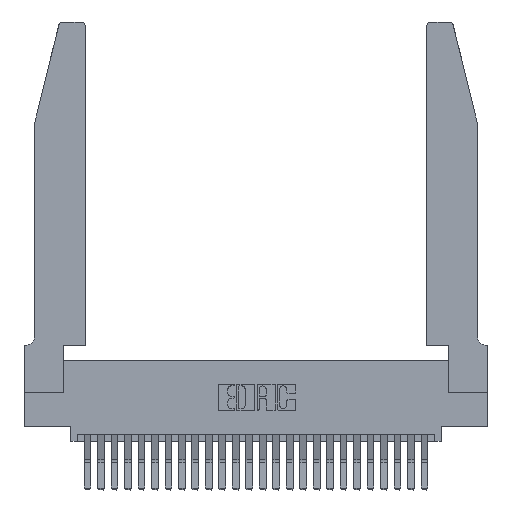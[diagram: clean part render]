
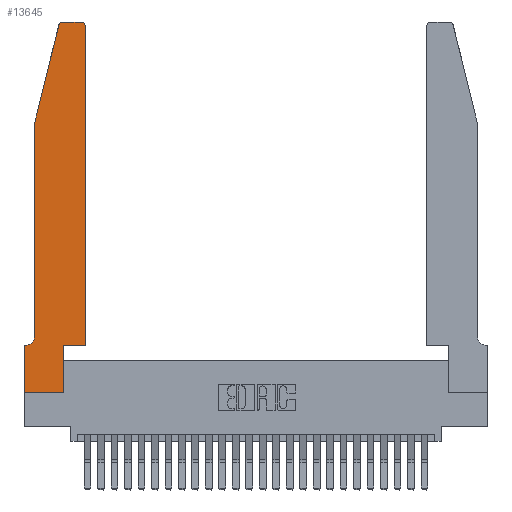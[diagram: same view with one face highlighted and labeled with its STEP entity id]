
A CAD part, top view. The second image highlights one B-rep face of the part: STEP entity #13645.
In plain terms, the highlighted planar face has unit normal (0, 0, 1).
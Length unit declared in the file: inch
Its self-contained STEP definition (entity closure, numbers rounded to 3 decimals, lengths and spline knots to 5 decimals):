
#191 = DIRECTION ( 'NONE',  ( -1., 0., 0. ) ) ;
#1623 = EDGE_CURVE ( 'NONE', #24799, #25691, #21712, .T. ) ;
#1647 = ORIENTED_EDGE ( 'NONE', *, *, #10541, .T. ) ;
#2577 = EDGE_CURVE ( 'NONE', #8014, #25782, #20995, .T. ) ;
#3032 = LINE ( 'NONE', #21042, #5004 ) ;
#3090 = CARTESIAN_POINT ( 'NONE',  ( 0.4505, 0.35, 0.37 ) ) ;
#3156 = EDGE_CURVE ( 'NONE', #8851, #26485, #5602, .T. ) ;
#3496 = DIRECTION ( 'NONE',  ( 1., 0., 0. ) ) ;
#3728 = VERTEX_POINT ( 'NONE', #27274 ) ;
#3862 = ORIENTED_EDGE ( 'NONE', *, *, #1623, .T. ) ;
#4601 = VECTOR ( 'NONE', #14679, 39.37008 ) ;
#4618 = CARTESIAN_POINT ( 'NONE',  ( 0.0055, 0.42, 0.37 ) ) ;
#5004 = VECTOR ( 'NONE', #8259, 39.37008 ) ;
#5112 = CARTESIAN_POINT ( 'NONE',  ( 0.2605, 2.75, 0.37 ) ) ;
#5154 = CARTESIAN_POINT ( 'NONE',  ( 0.0755, 2., 0.37 ) ) ;
#5415 = AXIS2_PLACEMENT_3D ( 'NONE', #16167, #5652, #9706 ) ;
#5602 = CIRCLE ( 'NONE', #13974, 0.07 ) ;
#5652 = DIRECTION ( 'NONE',  ( 0., 0., 1. ) ) ;
#5722 = CARTESIAN_POINT ( 'NONE',  ( 0.0755, 2., 0.37 ) ) ;
#5994 = CARTESIAN_POINT ( 'NONE',  ( 0., 0.35, 0.37 ) ) ;
#7004 = VECTOR ( 'NONE', #8012, 39.37008 ) ;
#7296 = EDGE_CURVE ( 'NONE', #27507, #11293, #3032, .T. ) ;
#7310 = CARTESIAN_POINT ( 'NONE',  ( 0.4205, 2.75, 0.37 ) ) ;
#7410 = DIRECTION ( 'NONE',  ( -0.239, -0.971, 0. ) ) ;
#8012 = DIRECTION ( 'NONE',  ( -1., 0., 0. ) ) ;
#8014 = VERTEX_POINT ( 'NONE', #7310 ) ;
#8026 = CARTESIAN_POINT ( 'NONE',  ( 0.0755, 2., 0.37 ) ) ;
#8071 = EDGE_CURVE ( 'NONE', #26485, #24799, #8670, .T. ) ;
#8141 = DIRECTION ( 'NONE',  ( 0., 1., 0. ) ) ;
#8259 = DIRECTION ( 'NONE',  ( 1., 0., 0. ) ) ;
#8312 = VECTOR ( 'NONE', #21281, 39.37008 ) ;
#8501 = CARTESIAN_POINT ( 'NONE',  ( 0., 0., 0.37 ) ) ;
#8670 = LINE ( 'NONE', #16443, #7004 ) ;
#8851 = VERTEX_POINT ( 'NONE', #23592 ) ;
#9061 = EDGE_CURVE ( 'NONE', #16507, #8851, #17365, .T. ) ;
#9536 = ORIENTED_EDGE ( 'NONE', *, *, #7296, .T. ) ;
#9549 = DIRECTION ( 'NONE',  ( 0., 1., 0. ) ) ;
#9706 = DIRECTION ( 'NONE',  ( 1., 0., 0. ) ) ;
#9871 = CARTESIAN_POINT ( 'NONE',  ( 0.4505, 2.72, 0.37 ) ) ;
#9877 = DIRECTION ( 'NONE',  ( 0., 0., 1. ) ) ;
#10463 = CARTESIAN_POINT ( 'NONE',  ( 0., 0., 0.37 ) ) ;
#10541 = EDGE_CURVE ( 'NONE', #11293, #24097, #25851, .T. ) ;
#11027 = ORIENTED_EDGE ( 'NONE', *, *, #16321, .T. ) ;
#11293 = VERTEX_POINT ( 'NONE', #25905 ) ;
#11529 = CARTESIAN_POINT ( 'NONE',  ( 0., 0., 0.37 ) ) ;
#12770 = EDGE_CURVE ( 'NONE', #24097, #8014, #15247, .T. ) ;
#13645 = ADVANCED_FACE ( 'NONE', ( #17851 ), #24749, .T. ) ;
#13974 = AXIS2_PLACEMENT_3D ( 'NONE', #4618, #17377, #191 ) ;
#14679 = DIRECTION ( 'NONE',  ( 0., -1., 0. ) ) ;
#15247 = CIRCLE ( 'NONE', #5415, 0.03 ) ;
#15413 = EDGE_LOOP ( 'NONE', ( #21035, #11027, #22888, #17339, #23902, #17139, #3862, #18591, #20110, #9536, #1647, #23882 ) ) ;
#16167 = CARTESIAN_POINT ( 'NONE',  ( 0.4205, 2.72, 0.37 ) ) ;
#16321 = EDGE_CURVE ( 'NONE', #25782, #16988, #19688, .T. ) ;
#16334 = CARTESIAN_POINT ( 'NONE',  ( 0., 0.35, 0.37 ) ) ;
#16443 = CARTESIAN_POINT ( 'NONE',  ( 0.0755, 0.35, 0.37 ) ) ;
#16507 = VERTEX_POINT ( 'NONE', #8026 ) ;
#16988 = VERTEX_POINT ( 'NONE', #22201 ) ;
#17003 = DIRECTION ( 'NONE',  ( 0., -1., 0. ) ) ;
#17102 = DIRECTION ( 'NONE',  ( 0., 0., 1. ) ) ;
#17139 = ORIENTED_EDGE ( 'NONE', *, *, #8071, .T. ) ;
#17339 = ORIENTED_EDGE ( 'NONE', *, *, #9061, .T. ) ;
#17363 = AXIS2_PLACEMENT_3D ( 'NONE', #16334, #9877, #3496 ) ;
#17365 = LINE ( 'NONE', #5722, #4601 ) ;
#17377 = DIRECTION ( 'NONE',  ( 0., 0., -1. ) ) ;
#17506 = VECTOR ( 'NONE', #7410, 39.37008 ) ;
#17851 = FACE_OUTER_BOUND ( 'NONE', #15413, .T. ) ;
#18591 = ORIENTED_EDGE ( 'NONE', *, *, #23031, .T. ) ;
#19032 = DIRECTION ( 'NONE',  ( 1., 0., 0. ) ) ;
#19242 = AXIS2_PLACEMENT_3D ( 'NONE', #21348, #17102, #19032 ) ;
#19688 = CIRCLE ( 'NONE', #19242, 0.03 ) ;
#19974 = LINE ( 'NONE', #27182, #20309 ) ;
#20110 = ORIENTED_EDGE ( 'NONE', *, *, #25981, .T. ) ;
#20244 = VECTOR ( 'NONE', #9549, 39.37008 ) ;
#20309 = VECTOR ( 'NONE', #8141, 39.37008 ) ;
#20372 = EDGE_CURVE ( 'NONE', #16988, #16507, #26743, .T. ) ;
#20995 = LINE ( 'NONE', #5112, #23967 ) ;
#21035 = ORIENTED_EDGE ( 'NONE', *, *, #2577, .T. ) ;
#21042 = CARTESIAN_POINT ( 'NONE',  ( 0.4505, 0.35, 0.37 ) ) ;
#21281 = DIRECTION ( 'NONE',  ( 1., 0., 0. ) ) ;
#21348 = CARTESIAN_POINT ( 'NONE',  ( 0.284, 2.72, 0.37 ) ) ;
#21712 = LINE ( 'NONE', #10463, #27008 ) ;
#22201 = CARTESIAN_POINT ( 'NONE',  ( 0.25487, 2.72718, 0.37 ) ) ;
#22577 = CARTESIAN_POINT ( 'NONE',  ( 0.0055, 0.35, 0.37 ) ) ;
#22888 = ORIENTED_EDGE ( 'NONE', *, *, #20372, .T. ) ;
#23031 = EDGE_CURVE ( 'NONE', #25691, #3728, #27268, .T. ) ;
#23592 = CARTESIAN_POINT ( 'NONE',  ( 0.0755, 0.42, 0.37 ) ) ;
#23882 = ORIENTED_EDGE ( 'NONE', *, *, #12770, .T. ) ;
#23902 = ORIENTED_EDGE ( 'NONE', *, *, #3156, .T. ) ;
#23967 = VECTOR ( 'NONE', #24408, 39.37008 ) ;
#24097 = VERTEX_POINT ( 'NONE', #9871 ) ;
#24408 = DIRECTION ( 'NONE',  ( -1., 0., 0. ) ) ;
#24427 = CARTESIAN_POINT ( 'NONE',  ( 0.284, 2.75, 0.37 ) ) ;
#24749 = PLANE ( 'NONE',  #17363 ) ;
#24799 = VERTEX_POINT ( 'NONE', #5994 ) ;
#25691 = VERTEX_POINT ( 'NONE', #11529 ) ;
#25782 = VERTEX_POINT ( 'NONE', #24427 ) ;
#25851 = LINE ( 'NONE', #3090, #20244 ) ;
#25905 = CARTESIAN_POINT ( 'NONE',  ( 0.4505, 0.35, 0.37 ) ) ;
#25981 = EDGE_CURVE ( 'NONE', #3728, #27507, #19974, .T. ) ;
#26485 = VERTEX_POINT ( 'NONE', #22577 ) ;
#26709 = CARTESIAN_POINT ( 'NONE',  ( 0.2865, 0.35, 0.37 ) ) ;
#26743 = LINE ( 'NONE', #5154, #17506 ) ;
#27008 = VECTOR ( 'NONE', #17003, 39.37008 ) ;
#27182 = CARTESIAN_POINT ( 'NONE',  ( 0.2865, 0.35, 0.37 ) ) ;
#27268 = LINE ( 'NONE', #8501, #8312 ) ;
#27274 = CARTESIAN_POINT ( 'NONE',  ( 0.2865, 0., 0.37 ) ) ;
#27507 = VERTEX_POINT ( 'NONE', #26709 ) ;
